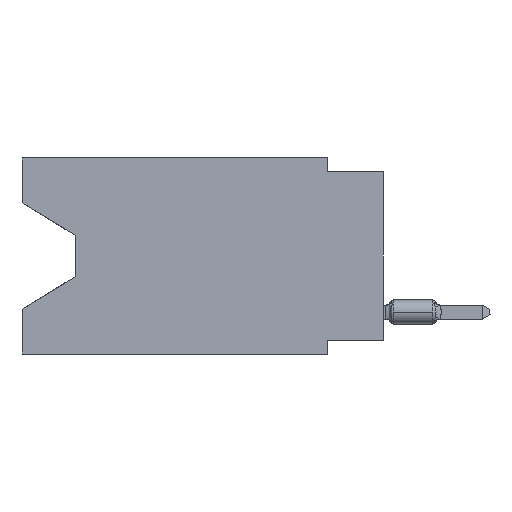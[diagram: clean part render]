
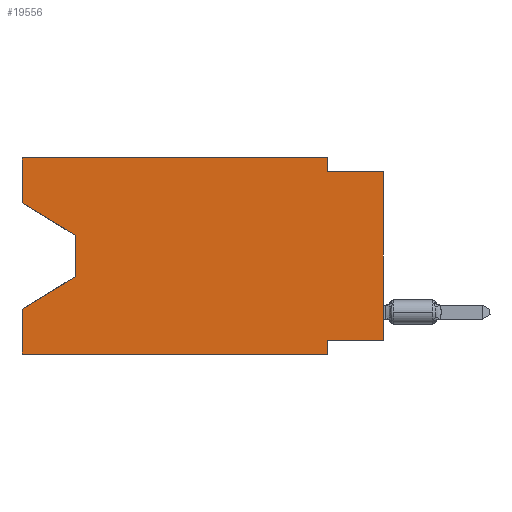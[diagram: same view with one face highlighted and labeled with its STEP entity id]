
A CAD part, left-side view. The second image highlights one B-rep face of the part: STEP entity #19556.
In plain terms, the highlighted planar face has unit normal (-1, 0, 0).
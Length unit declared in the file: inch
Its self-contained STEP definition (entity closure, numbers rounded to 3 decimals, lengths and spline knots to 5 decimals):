
#509 = VERTEX_POINT ( 'NONE', #10241 ) ;
#5003 = VECTOR ( 'NONE', #62980, 39.37008 ) ;
#5629 = CARTESIAN_POINT ( 'NONE',  ( 0., 0.1, -0.35 ) ) ;
#6072 = ORIENTED_EDGE ( 'NONE', *, *, #110667, .F. ) ;
#6293 = LINE ( 'NONE', #24820, #90714 ) ;
#6423 = CARTESIAN_POINT ( 'NONE',  ( 0., 0.1, -0.325 ) ) ;
#6712 = DIRECTION ( 'NONE',  ( 0., 1., 0. ) ) ;
#6774 = DIRECTION ( 'NONE',  ( 0., 0., -1. ) ) ;
#9071 = EDGE_CURVE ( 'NONE', #104169, #19394, #57487, .T. ) ;
#10155 = LINE ( 'NONE', #62977, #94567 ) ;
#10241 = CARTESIAN_POINT ( 'NONE',  ( 0., 0.645, -0.08025 ) ) ;
#10445 = VERTEX_POINT ( 'NONE', #42317 ) ;
#11144 = VECTOR ( 'NONE', #74957, 39.37008 ) ;
#12253 = DIRECTION ( 'NONE',  ( 0., 0.855, -0.519 ) ) ;
#12381 = EDGE_CURVE ( 'NONE', #51489, #93121, #6293, .T. ) ;
#13713 = DIRECTION ( 'NONE',  ( 0., 0., 1. ) ) ;
#14291 = VECTOR ( 'NONE', #57086, 39.37008 ) ;
#15482 = EDGE_CURVE ( 'NONE', #509, #10445, #10155, .T. ) ;
#19394 = VERTEX_POINT ( 'NONE', #91497 ) ;
#19556 = ADVANCED_FACE ( 'NONE', ( #114193 ), #61359, .F. ) ;
#19773 = EDGE_CURVE ( 'NONE', #509, #50810, #73960, .T. ) ;
#20191 = EDGE_CURVE ( 'NONE', #67680, #107330, #56389, .T. ) ;
#20808 = EDGE_CURVE ( 'NONE', #51489, #107330, #57952, .T. ) ;
#23933 = VERTEX_POINT ( 'NONE', #6423 ) ;
#24343 = CARTESIAN_POINT ( 'NONE',  ( 0., 0.645, 0. ) ) ;
#24820 = CARTESIAN_POINT ( 'NONE',  ( 0., 0.645, -0.35 ) ) ;
#25910 = DIRECTION ( 'NONE',  ( 1., 0., 0. ) ) ;
#26360 = VERTEX_POINT ( 'NONE', #100700 ) ;
#27200 = ORIENTED_EDGE ( 'NONE', *, *, #20191, .T. ) ;
#29461 = ORIENTED_EDGE ( 'NONE', *, *, #61744, .F. ) ;
#30203 = CARTESIAN_POINT ( 'NONE',  ( 0., 0., -0.025 ) ) ;
#34122 = ORIENTED_EDGE ( 'NONE', *, *, #43140, .F. ) ;
#34243 = ORIENTED_EDGE ( 'NONE', *, *, #15482, .T. ) ;
#35237 = DIRECTION ( 'NONE',  ( 0., -1., 0. ) ) ;
#35678 = CARTESIAN_POINT ( 'NONE',  ( 0., 0.55, -0.138 ) ) ;
#36096 = ORIENTED_EDGE ( 'NONE', *, *, #78952, .T. ) ;
#36344 = DIRECTION ( 'NONE',  ( 0., 0., -1. ) ) ;
#39862 = VECTOR ( 'NONE', #61511, 39.37008 ) ;
#41092 = DIRECTION ( 'NONE',  ( 0., 0., 1. ) ) ;
#41768 = CARTESIAN_POINT ( 'NONE',  ( 0., 0.1, -0.025 ) ) ;
#42099 = CARTESIAN_POINT ( 'NONE',  ( 0., 0., -0.325 ) ) ;
#42317 = CARTESIAN_POINT ( 'NONE',  ( 0., 0.55, -0.138 ) ) ;
#43140 = EDGE_CURVE ( 'NONE', #109528, #23933, #67718, .T. ) ;
#44382 = LINE ( 'NONE', #35678, #5003 ) ;
#45530 = DIRECTION ( 'NONE',  ( 0., -0.855, -0.519 ) ) ;
#46936 = VECTOR ( 'NONE', #6712, 39.37008 ) ;
#49687 = LINE ( 'NONE', #56704, #51568 ) ;
#49923 = LINE ( 'NONE', #24343, #86943 ) ;
#50810 = VERTEX_POINT ( 'NONE', #73818 ) ;
#51067 = EDGE_CURVE ( 'NONE', #26360, #104169, #86504, .T. ) ;
#51489 = VERTEX_POINT ( 'NONE', #104352 ) ;
#51568 = VECTOR ( 'NONE', #13713, 39.37008 ) ;
#55142 = ORIENTED_EDGE ( 'NONE', *, *, #20808, .F. ) ;
#56389 = LINE ( 'NONE', #83682, #77455 ) ;
#56704 = CARTESIAN_POINT ( 'NONE',  ( 0., 0., 0. ) ) ;
#57086 = DIRECTION ( 'NONE',  ( 0., 0., 1. ) ) ;
#57487 = LINE ( 'NONE', #30203, #11144 ) ;
#57905 = LINE ( 'NONE', #5629, #81426 ) ;
#57952 = LINE ( 'NONE', #85237, #58969 ) ;
#58736 = CARTESIAN_POINT ( 'NONE',  ( 0., 0., -0.325 ) ) ;
#58969 = VECTOR ( 'NONE', #41092, 39.37008 ) ;
#60280 = ORIENTED_EDGE ( 'NONE', *, *, #9071, .F. ) ;
#61359 = PLANE ( 'NONE',  #103325 ) ;
#61511 = DIRECTION ( 'NONE',  ( 0., 0., -1. ) ) ;
#61548 = ORIENTED_EDGE ( 'NONE', *, *, #51067, .F. ) ;
#61744 = EDGE_CURVE ( 'NONE', #50810, #26360, #49923, .T. ) ;
#62977 = CARTESIAN_POINT ( 'NONE',  ( 0., 0.645, -0.08025 ) ) ;
#62980 = DIRECTION ( 'NONE',  ( 0., 0., -1. ) ) ;
#67497 = ORIENTED_EDGE ( 'NONE', *, *, #19773, .F. ) ;
#67680 = VERTEX_POINT ( 'NONE', #103612 ) ;
#67718 = LINE ( 'NONE', #42099, #46936 ) ;
#69088 = CARTESIAN_POINT ( 'NONE',  ( 0., 0.1, 0. ) ) ;
#70656 = CARTESIAN_POINT ( 'NONE',  ( 0., 0.645, 0. ) ) ;
#73818 = CARTESIAN_POINT ( 'NONE',  ( 0., 0.645, 0. ) ) ;
#73960 = LINE ( 'NONE', #109937, #14291 ) ;
#74957 = DIRECTION ( 'NONE',  ( 0., -1., 0. ) ) ;
#77455 = VECTOR ( 'NONE', #12253, 39.37008 ) ;
#78697 = EDGE_CURVE ( 'NONE', #109528, #19394, #49687, .T. ) ;
#78952 = EDGE_CURVE ( 'NONE', #10445, #67680, #44382, .T. ) ;
#81426 = VECTOR ( 'NONE', #6774, 39.37008 ) ;
#83682 = CARTESIAN_POINT ( 'NONE',  ( 0., 0.55, -0.212 ) ) ;
#84610 = CARTESIAN_POINT ( 'NONE',  ( 0., 0.1, -0.35 ) ) ;
#85237 = CARTESIAN_POINT ( 'NONE',  ( 0., 0.645, 0. ) ) ;
#86504 = LINE ( 'NONE', #69088, #39862 ) ;
#86943 = VECTOR ( 'NONE', #93505, 39.37008 ) ;
#90714 = VECTOR ( 'NONE', #35237, 39.37008 ) ;
#91497 = CARTESIAN_POINT ( 'NONE',  ( 0., 0., -0.025 ) ) ;
#93121 = VERTEX_POINT ( 'NONE', #84610 ) ;
#93505 = DIRECTION ( 'NONE',  ( 0., -1., 0. ) ) ;
#94567 = VECTOR ( 'NONE', #45530, 39.37008 ) ;
#99710 = CARTESIAN_POINT ( 'NONE',  ( 0., 0.645, -0.26975 ) ) ;
#100700 = CARTESIAN_POINT ( 'NONE',  ( 0., 0.1, 0. ) ) ;
#103325 = AXIS2_PLACEMENT_3D ( 'NONE', #70656, #25910, #36344 ) ;
#103612 = CARTESIAN_POINT ( 'NONE',  ( 0., 0.55, -0.212 ) ) ;
#104169 = VERTEX_POINT ( 'NONE', #41768 ) ;
#104352 = CARTESIAN_POINT ( 'NONE',  ( 0., 0.645, -0.35 ) ) ;
#106739 = ORIENTED_EDGE ( 'NONE', *, *, #12381, .T. ) ;
#107098 = ORIENTED_EDGE ( 'NONE', *, *, #78697, .T. ) ;
#107330 = VERTEX_POINT ( 'NONE', #99710 ) ;
#108665 = EDGE_LOOP ( 'NONE', ( #34243, #36096, #27200, #55142, #106739, #6072, #34122, #107098, #60280, #61548, #29461, #67497 ) ) ;
#109528 = VERTEX_POINT ( 'NONE', #58736 ) ;
#109937 = CARTESIAN_POINT ( 'NONE',  ( 0., 0.645, 0. ) ) ;
#110667 = EDGE_CURVE ( 'NONE', #23933, #93121, #57905, .T. ) ;
#114193 = FACE_OUTER_BOUND ( 'NONE', #108665, .T. ) ;
